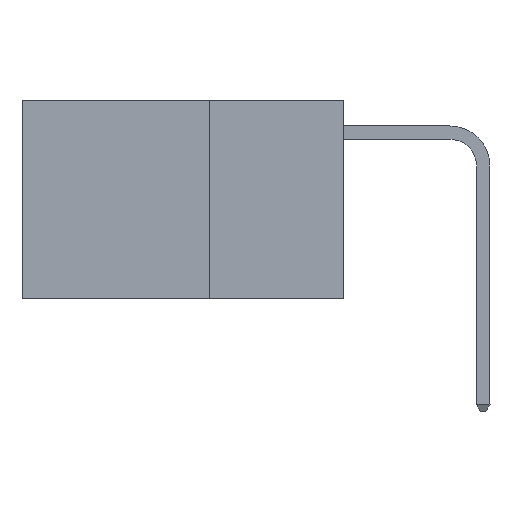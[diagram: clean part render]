
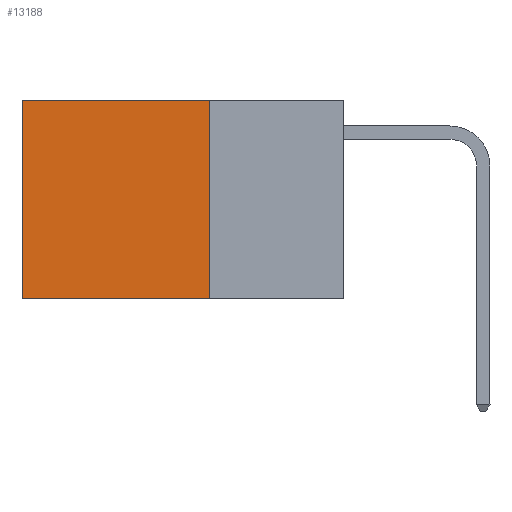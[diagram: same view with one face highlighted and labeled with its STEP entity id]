
A CAD part, left-side view. The second image highlights one B-rep face of the part: STEP entity #13188.
In plain terms, the highlighted planar face has unit normal (-1, 0, 0).
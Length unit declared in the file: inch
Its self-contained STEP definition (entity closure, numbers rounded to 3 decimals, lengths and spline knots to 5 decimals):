
#2 = EDGE_LOOP ( 'NONE', ( #7470, #1403, #4332, #8256 ) ) ;
#527 = LINE ( 'NONE', #6349, #12137 ) ;
#774 = LINE ( 'NONE', #12513, #2332 ) ;
#1403 = ORIENTED_EDGE ( 'NONE', *, *, #7734, .F. ) ;
#1714 = DIRECTION ( 'NONE',  ( 0., 0., -1. ) ) ;
#1993 = VERTEX_POINT ( 'NONE', #7207 ) ;
#2332 = VECTOR ( 'NONE', #11179, 39.37008 ) ;
#2979 = CARTESIAN_POINT ( 'NONE',  ( 0.2625, 0.6, 0. ) ) ;
#3169 = FACE_OUTER_BOUND ( 'NONE', #2, .T. ) ;
#3824 = VECTOR ( 'NONE', #16581, 39.37008 ) ;
#4332 = ORIENTED_EDGE ( 'NONE', *, *, #5394, .F. ) ;
#5394 = EDGE_CURVE ( 'NONE', #1993, #13373, #774, .T. ) ;
#6349 = CARTESIAN_POINT ( 'NONE',  ( 0.2625, 0.6, 0. ) ) ;
#7207 = CARTESIAN_POINT ( 'NONE',  ( 0.2625, 0.25, 0. ) ) ;
#7470 = ORIENTED_EDGE ( 'NONE', *, *, #10516, .T. ) ;
#7734 = EDGE_CURVE ( 'NONE', #13373, #16676, #11977, .T. ) ;
#7798 = DIRECTION ( 'NONE',  ( 0., 1., 0. ) ) ;
#8256 = ORIENTED_EDGE ( 'NONE', *, *, #17734, .T. ) ;
#8592 = VERTEX_POINT ( 'NONE', #2979 ) ;
#8979 = CARTESIAN_POINT ( 'NONE',  ( 0.2625, 0.25, 0. ) ) ;
#9048 = CARTESIAN_POINT ( 'NONE',  ( 0.2625, 0.25, -0.37 ) ) ;
#9072 = PLANE ( 'NONE',  #15832 ) ;
#9309 = LINE ( 'NONE', #12255, #3824 ) ;
#10516 = EDGE_CURVE ( 'NONE', #8592, #16676, #527, .T. ) ;
#11179 = DIRECTION ( 'NONE',  ( 0., 0., -1. ) ) ;
#11977 = LINE ( 'NONE', #9048, #14392 ) ;
#12137 = VECTOR ( 'NONE', #17918, 39.37008 ) ;
#12255 = CARTESIAN_POINT ( 'NONE',  ( 0.2625, 0.25, 0. ) ) ;
#12513 = CARTESIAN_POINT ( 'NONE',  ( 0.2625, 0.25, 0. ) ) ;
#13188 = ADVANCED_FACE ( 'NONE', ( #3169 ), #9072, .F. ) ;
#13373 = VERTEX_POINT ( 'NONE', #16706 ) ;
#14392 = VECTOR ( 'NONE', #7798, 39.37008 ) ;
#14762 = DIRECTION ( 'NONE',  ( 1., 0., 0. ) ) ;
#15832 = AXIS2_PLACEMENT_3D ( 'NONE', #8979, #14762, #1714 ) ;
#16581 = DIRECTION ( 'NONE',  ( 0., 1., 0. ) ) ;
#16676 = VERTEX_POINT ( 'NONE', #17350 ) ;
#16706 = CARTESIAN_POINT ( 'NONE',  ( 0.2625, 0.25, -0.37 ) ) ;
#17350 = CARTESIAN_POINT ( 'NONE',  ( 0.2625, 0.6, -0.37 ) ) ;
#17734 = EDGE_CURVE ( 'NONE', #1993, #8592, #9309, .T. ) ;
#17918 = DIRECTION ( 'NONE',  ( 0., 0., -1. ) ) ;
